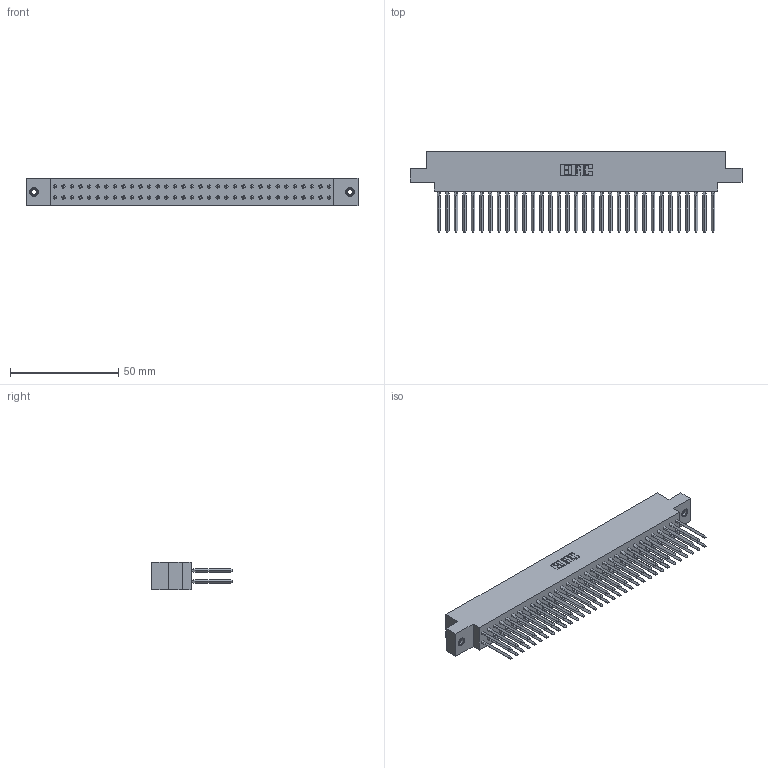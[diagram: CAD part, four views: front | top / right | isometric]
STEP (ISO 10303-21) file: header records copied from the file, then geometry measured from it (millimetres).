
FILE_DESCRIPTION (( 'STEP AP203' ), '1' );
FILE_NAME ('317-066-542-808.STEP', '2020-02-28T06:20:57', ( '' ), ( '' ), 'SwSTEP 2.0', 'SolidWorks 2016', '' );
FILE_SCHEMA (( 'CONFIG_CONTROL_DESIGN' ));
Length unit declared in the file: inch
Products named in the file (4): 317-290-003_542; 317-066-542-808; 345-250-001_345-250-003-102; 317 Part_.156 Dia - TI
Assembly tree (69 placements, depth 2):
  317-066-542-808
    317 Part_.156 Dia - TI
    317-290-003_542  x66
    345-250-001_345-250-003-102  x2
Bounding box: 153.47 x 37.34 x 12.7 mm (x, y, z)
Volume: 24838.7 mm3; surface area: 34274.3 mm2
Topology: 69 solids, 69 shells, 3924 faces, 10971 edges, 6998 vertices
Faces by surface type: plane 3126, cylinder 518, bspline 264, cone 12, torus 4
Entity records: 49160 total; most frequent: CARTESIAN_POINT 8796, ORIENTED_EDGE 8452, DIRECTION 7164, EDGE_CURVE 4226, VECTOR 4036, LINE 4036, VERTEX_POINT 2808, AXIS2_PLACEMENT_3D 1564
